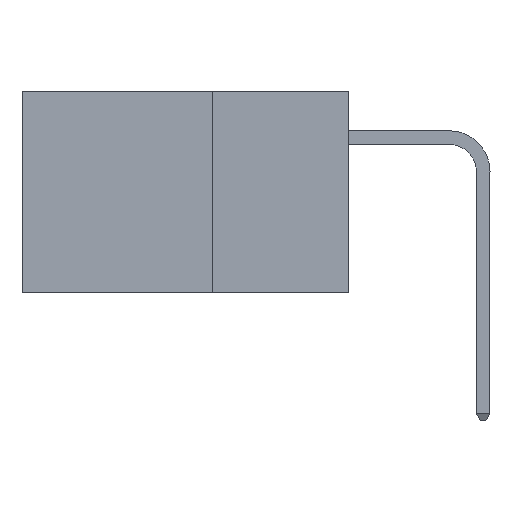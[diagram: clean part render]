
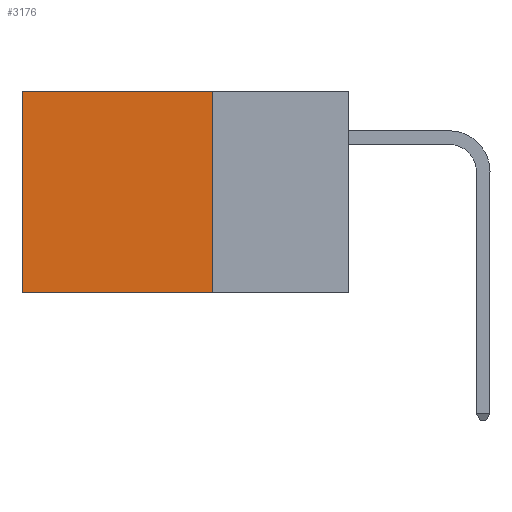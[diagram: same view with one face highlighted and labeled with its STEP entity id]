
A CAD part, left-side view. The second image highlights one B-rep face of the part: STEP entity #3176.
In plain terms, the highlighted planar face has unit normal (-1, 0, 0).
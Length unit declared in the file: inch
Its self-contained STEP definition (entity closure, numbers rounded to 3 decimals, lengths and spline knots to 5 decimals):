
#350 = DIRECTION ( 'NONE',  ( 0., 1., 0. ) ) ;
#565 = ORIENTED_EDGE ( 'NONE', *, *, #1505, .T. ) ;
#603 = ORIENTED_EDGE ( 'NONE', *, *, #1820, .F. ) ;
#945 = CARTESIAN_POINT ( 'NONE',  ( 0.2875, 0.25, -0.37 ) ) ;
#1227 = EDGE_CURVE ( 'NONE', #17626, #1873, #1575, .T. ) ;
#1505 = EDGE_CURVE ( 'NONE', #5831, #17626, #9692, .T. ) ;
#1575 = LINE ( 'NONE', #7412, #6382 ) ;
#1820 = EDGE_CURVE ( 'NONE', #19889, #1873, #13358, .T. ) ;
#1873 = VERTEX_POINT ( 'NONE', #11228 ) ;
#2249 = VECTOR ( 'NONE', #7481, 39.37008 ) ;
#3176 = ADVANCED_FACE ( 'NONE', ( #17284 ), #4038, .F. ) ;
#3874 = CARTESIAN_POINT ( 'NONE',  ( 0.2875, 0.25, 0. ) ) ;
#4038 = PLANE ( 'NONE',  #20291 ) ;
#4420 = ORIENTED_EDGE ( 'NONE', *, *, #1227, .T. ) ;
#4968 = VECTOR ( 'NONE', #7979, 39.37008 ) ;
#5831 = VERTEX_POINT ( 'NONE', #18233 ) ;
#5832 = DIRECTION ( 'NONE',  ( 1., 0., 0. ) ) ;
#6382 = VECTOR ( 'NONE', #15895, 39.37008 ) ;
#7122 = CARTESIAN_POINT ( 'NONE',  ( 0.2875, 0.6, 0. ) ) ;
#7412 = CARTESIAN_POINT ( 'NONE',  ( 0.2875, 0.6, 0. ) ) ;
#7481 = DIRECTION ( 'NONE',  ( 0., 0., -1. ) ) ;
#7979 = DIRECTION ( 'NONE',  ( 0., 1., 0. ) ) ;
#9325 = CARTESIAN_POINT ( 'NONE',  ( 0.2875, 0.25, -0.37 ) ) ;
#9692 = LINE ( 'NONE', #3874, #4968 ) ;
#11228 = CARTESIAN_POINT ( 'NONE',  ( 0.2875, 0.6, -0.37 ) ) ;
#11618 = ORIENTED_EDGE ( 'NONE', *, *, #13762, .F. ) ;
#13358 = LINE ( 'NONE', #9325, #21738 ) ;
#13762 = EDGE_CURVE ( 'NONE', #5831, #19889, #19005, .T. ) ;
#14401 = CARTESIAN_POINT ( 'NONE',  ( 0.2875, 0.25, 0. ) ) ;
#15895 = DIRECTION ( 'NONE',  ( 0., 0., -1. ) ) ;
#17284 = FACE_OUTER_BOUND ( 'NONE', #20304, .T. ) ;
#17626 = VERTEX_POINT ( 'NONE', #7122 ) ;
#17654 = CARTESIAN_POINT ( 'NONE',  ( 0.2875, 0.25, 0. ) ) ;
#17825 = DIRECTION ( 'NONE',  ( 0., 0., -1. ) ) ;
#18233 = CARTESIAN_POINT ( 'NONE',  ( 0.2875, 0.25, 0. ) ) ;
#19005 = LINE ( 'NONE', #17654, #2249 ) ;
#19889 = VERTEX_POINT ( 'NONE', #945 ) ;
#20291 = AXIS2_PLACEMENT_3D ( 'NONE', #14401, #5832, #17825 ) ;
#20304 = EDGE_LOOP ( 'NONE', ( #4420, #603, #11618, #565 ) ) ;
#21738 = VECTOR ( 'NONE', #350, 39.37008 ) ;
